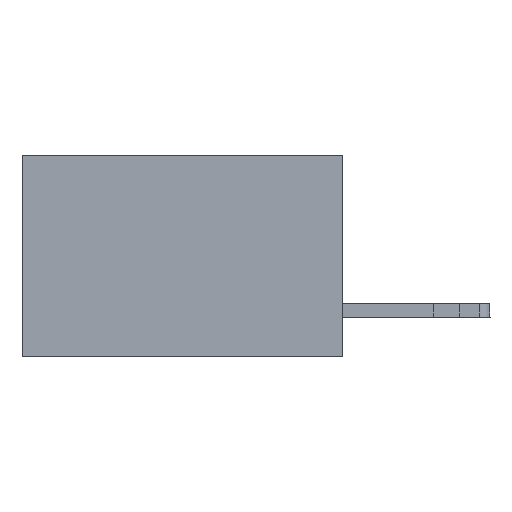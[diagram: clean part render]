
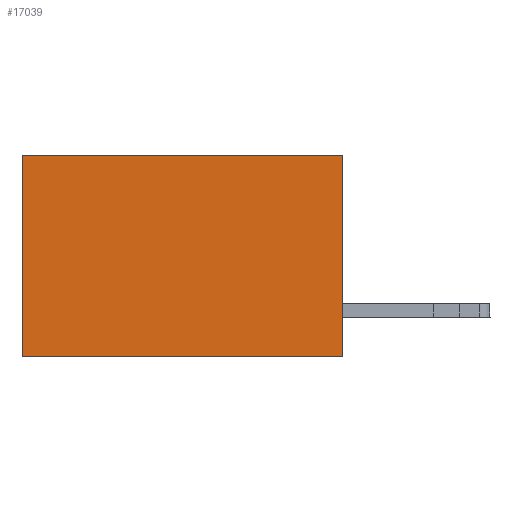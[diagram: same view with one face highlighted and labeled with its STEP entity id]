
A CAD part, left-side view. The second image highlights one B-rep face of the part: STEP entity #17039.
In plain terms, the highlighted planar face has unit normal (-1, 0, 0).
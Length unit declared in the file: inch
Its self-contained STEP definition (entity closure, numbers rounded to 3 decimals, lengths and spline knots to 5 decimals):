
#526 = LINE ( 'NONE', #7678, #9849 ) ;
#1113 = LINE ( 'NONE', #7693, #26397 ) ;
#3212 = CARTESIAN_POINT ( 'NONE',  ( 0.277, 0.59, 0. ) ) ;
#3509 = VERTEX_POINT ( 'NONE', #7131 ) ;
#3723 = CARTESIAN_POINT ( 'NONE',  ( 0.277, 0., -0.37 ) ) ;
#5155 = DIRECTION ( 'NONE',  ( 0., 0., -1. ) ) ;
#7131 = CARTESIAN_POINT ( 'NONE',  ( 0.277, 0.59, -0.37 ) ) ;
#7678 = CARTESIAN_POINT ( 'NONE',  ( 0.277, 0., 0. ) ) ;
#7693 = CARTESIAN_POINT ( 'NONE',  ( 0.277, 0.59, -0.37 ) ) ;
#8458 = VERTEX_POINT ( 'NONE', #3212 ) ;
#8796 = PLANE ( 'NONE',  #25452 ) ;
#9362 = LINE ( 'NONE', #27920, #16278 ) ;
#9849 = VECTOR ( 'NONE', #10067, 39.37008 ) ;
#10067 = DIRECTION ( 'NONE',  ( 0., 1., 0. ) ) ;
#11248 = ORIENTED_EDGE ( 'NONE', *, *, #27871, .T. ) ;
#12000 = CARTESIAN_POINT ( 'NONE',  ( 0.277, 0., -0.37 ) ) ;
#12276 = LINE ( 'NONE', #12000, #16111 ) ;
#12850 = DIRECTION ( 'NONE',  ( 0., 0., -1. ) ) ;
#12886 = EDGE_CURVE ( 'NONE', #21693, #3509, #9362, .T. ) ;
#16111 = VECTOR ( 'NONE', #23360, 39.37008 ) ;
#16278 = VECTOR ( 'NONE', #21017, 39.37008 ) ;
#17039 = ADVANCED_FACE ( 'NONE', ( #22399 ), #8796, .F. ) ;
#17306 = ORIENTED_EDGE ( 'NONE', *, *, #12886, .F. ) ;
#17868 = VERTEX_POINT ( 'NONE', #26942 ) ;
#18160 = EDGE_LOOP ( 'NONE', ( #11248, #17306, #20565, #21611 ) ) ;
#20299 = EDGE_CURVE ( 'NONE', #17868, #8458, #526, .T. ) ;
#20565 = ORIENTED_EDGE ( 'NONE', *, *, #20840, .F. ) ;
#20840 = EDGE_CURVE ( 'NONE', #17868, #21693, #12276, .T. ) ;
#21017 = DIRECTION ( 'NONE',  ( 0., 1., 0. ) ) ;
#21611 = ORIENTED_EDGE ( 'NONE', *, *, #20299, .T. ) ;
#21693 = VERTEX_POINT ( 'NONE', #25973 ) ;
#22399 = FACE_OUTER_BOUND ( 'NONE', #18160, .T. ) ;
#23360 = DIRECTION ( 'NONE',  ( 0., 0., -1. ) ) ;
#24213 = DIRECTION ( 'NONE',  ( 1., 0., 0. ) ) ;
#25452 = AXIS2_PLACEMENT_3D ( 'NONE', #3723, #24213, #12850 ) ;
#25973 = CARTESIAN_POINT ( 'NONE',  ( 0.277, 0., -0.37 ) ) ;
#26397 = VECTOR ( 'NONE', #5155, 39.37008 ) ;
#26942 = CARTESIAN_POINT ( 'NONE',  ( 0.277, 0., 0. ) ) ;
#27871 = EDGE_CURVE ( 'NONE', #8458, #3509, #1113, .T. ) ;
#27920 = CARTESIAN_POINT ( 'NONE',  ( 0.277, 0., -0.37 ) ) ;
